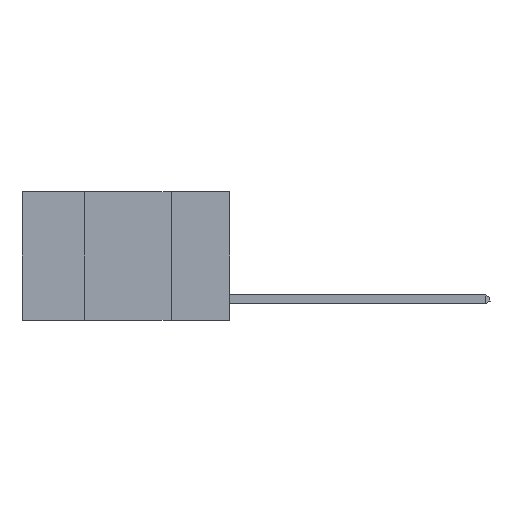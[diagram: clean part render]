
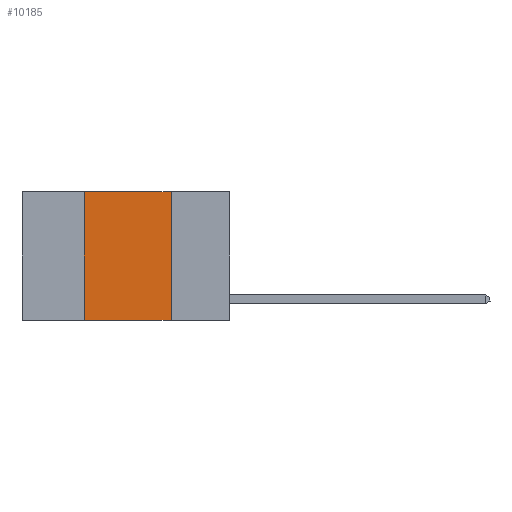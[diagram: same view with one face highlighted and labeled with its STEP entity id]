
A CAD part, left-side view. The second image highlights one B-rep face of the part: STEP entity #10185.
In plain terms, the highlighted planar face has unit normal (-1, 0, 0).
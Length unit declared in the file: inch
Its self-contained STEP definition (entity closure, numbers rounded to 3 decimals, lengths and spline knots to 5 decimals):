
#8 = EDGE_CURVE ( 'NONE', #5346, #11417, #8033, .T. ) ;
#34 = CARTESIAN_POINT ( 'NONE',  ( 0., 0.6, 0. ) ) ;
#246 = VERTEX_POINT ( 'NONE', #8953 ) ;
#1928 = DIRECTION ( 'NONE',  ( 0., 0., -1. ) ) ;
#2863 = EDGE_CURVE ( 'NONE', #11417, #246, #10445, .T. ) ;
#3243 = VECTOR ( 'NONE', #11535, 39.37008 ) ;
#3309 = CARTESIAN_POINT ( 'NONE',  ( 0., 0.6, -0.37 ) ) ;
#3757 = DIRECTION ( 'NONE',  ( 0., -1., 0. ) ) ;
#4071 = DIRECTION ( 'NONE',  ( 0., -1., 0. ) ) ;
#4111 = CARTESIAN_POINT ( 'NONE',  ( 0., 0.42, 0. ) ) ;
#4354 = ORIENTED_EDGE ( 'NONE', *, *, #8, .F. ) ;
#4372 = VECTOR ( 'NONE', #4071, 39.37008 ) ;
#4503 = ORIENTED_EDGE ( 'NONE', *, *, #2863, .F. ) ;
#5346 = VERTEX_POINT ( 'NONE', #4111 ) ;
#5452 = CARTESIAN_POINT ( 'NONE',  ( 0., 0.42, -0.37 ) ) ;
#6003 = FACE_OUTER_BOUND ( 'NONE', #12954, .T. ) ;
#6463 = EDGE_CURVE ( 'NONE', #12376, #5346, #12550, .T. ) ;
#6870 = DIRECTION ( 'NONE',  ( 1., 0., 0. ) ) ;
#7514 = CARTESIAN_POINT ( 'NONE',  ( 0., 0.42, 0. ) ) ;
#8033 = LINE ( 'NONE', #12811, #11759 ) ;
#8554 = CARTESIAN_POINT ( 'NONE',  ( 0., 0.17, 0. ) ) ;
#8692 = AXIS2_PLACEMENT_3D ( 'NONE', #34, #6870, #1928 ) ;
#8744 = DIRECTION ( 'NONE',  ( 0., 0., -1. ) ) ;
#8953 = CARTESIAN_POINT ( 'NONE',  ( 0., 0.17, -0.37 ) ) ;
#9063 = PLANE ( 'NONE',  #8692 ) ;
#9516 = CARTESIAN_POINT ( 'NONE',  ( 0., 0.17, 0. ) ) ;
#9982 = ORIENTED_EDGE ( 'NONE', *, *, #10661, .T. ) ;
#10185 = ADVANCED_FACE ( 'NONE', ( #6003 ), #9063, .F. ) ;
#10344 = VECTOR ( 'NONE', #8744, 39.37008 ) ;
#10445 = LINE ( 'NONE', #8554, #10344 ) ;
#10661 = EDGE_CURVE ( 'NONE', #12376, #246, #12140, .T. ) ;
#11083 = ORIENTED_EDGE ( 'NONE', *, *, #6463, .F. ) ;
#11417 = VERTEX_POINT ( 'NONE', #9516 ) ;
#11535 = DIRECTION ( 'NONE',  ( 0., 0., 1. ) ) ;
#11759 = VECTOR ( 'NONE', #3757, 39.37008 ) ;
#12140 = LINE ( 'NONE', #3309, #4372 ) ;
#12376 = VERTEX_POINT ( 'NONE', #5452 ) ;
#12550 = LINE ( 'NONE', #7514, #3243 ) ;
#12811 = CARTESIAN_POINT ( 'NONE',  ( 0., 0.6, 0. ) ) ;
#12954 = EDGE_LOOP ( 'NONE', ( #4503, #4354, #11083, #9982 ) ) ;
